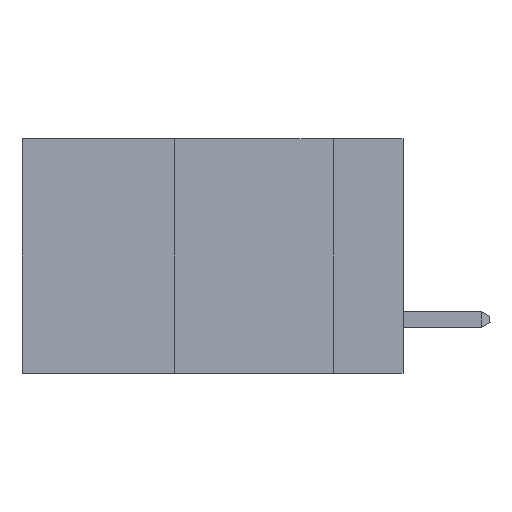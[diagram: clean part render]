
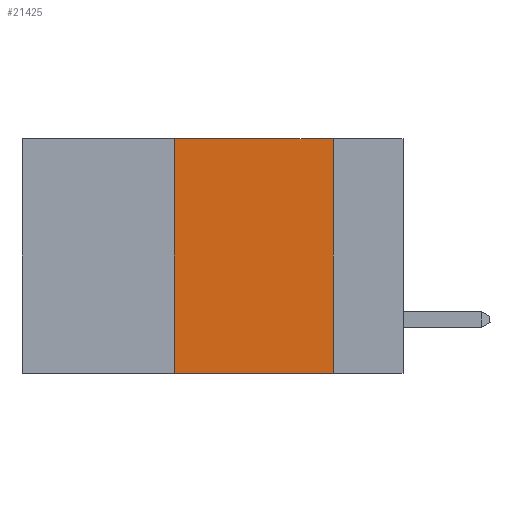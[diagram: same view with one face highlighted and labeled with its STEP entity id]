
A CAD part, left-side view. The second image highlights one B-rep face of the part: STEP entity #21425.
In plain terms, the highlighted planar face has unit normal (-1, 0, 0).
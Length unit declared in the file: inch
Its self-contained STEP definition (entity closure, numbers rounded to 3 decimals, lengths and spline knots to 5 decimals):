
#804 = LINE ( 'NONE', #48324, #30800 ) ;
#2694 = DIRECTION ( 'NONE',  ( 0., 0., -1. ) ) ;
#4091 = LINE ( 'NONE', #30993, #13079 ) ;
#6297 = CARTESIAN_POINT ( 'NONE',  ( 0., 0.36, -0.37 ) ) ;
#6637 = VERTEX_POINT ( 'NONE', #6297 ) ;
#9237 = VERTEX_POINT ( 'NONE', #23017 ) ;
#9293 = LINE ( 'NONE', #42395, #11704 ) ;
#9972 = EDGE_CURVE ( 'NONE', #19945, #35647, #4091, .T. ) ;
#10229 = CARTESIAN_POINT ( 'NONE',  ( 0., 0.11, 0. ) ) ;
#11704 = VECTOR ( 'NONE', #15233, 39.37008 ) ;
#13079 = VECTOR ( 'NONE', #39046, 39.37008 ) ;
#13133 = EDGE_CURVE ( 'NONE', #6637, #19945, #804, .T. ) ;
#14404 = EDGE_CURVE ( 'NONE', #35647, #9237, #40862, .T. ) ;
#14637 = EDGE_LOOP ( 'NONE', ( #26717, #46344, #33234, #18189 ) ) ;
#15233 = DIRECTION ( 'NONE',  ( 0., -1., 0. ) ) ;
#18189 = ORIENTED_EDGE ( 'NONE', *, *, #30617, .T. ) ;
#18473 = PLANE ( 'NONE',  #37638 ) ;
#19945 = VERTEX_POINT ( 'NONE', #43321 ) ;
#21425 = ADVANCED_FACE ( 'NONE', ( #24506 ), #18473, .F. ) ;
#22323 = DIRECTION ( 'NONE',  ( 0., 0., -1. ) ) ;
#23017 = CARTESIAN_POINT ( 'NONE',  ( 0., 0.11, -0.37 ) ) ;
#24506 = FACE_OUTER_BOUND ( 'NONE', #14637, .T. ) ;
#26717 = ORIENTED_EDGE ( 'NONE', *, *, #14404, .F. ) ;
#27049 = VECTOR ( 'NONE', #2694, 39.37008 ) ;
#30617 = EDGE_CURVE ( 'NONE', #6637, #9237, #9293, .T. ) ;
#30800 = VECTOR ( 'NONE', #44292, 39.37008 ) ;
#30993 = CARTESIAN_POINT ( 'NONE',  ( 0., 0.6, 0. ) ) ;
#33234 = ORIENTED_EDGE ( 'NONE', *, *, #13133, .F. ) ;
#33893 = DIRECTION ( 'NONE',  ( 1., 0., 0. ) ) ;
#35647 = VERTEX_POINT ( 'NONE', #48845 ) ;
#37638 = AXIS2_PLACEMENT_3D ( 'NONE', #45314, #33893, #22323 ) ;
#39046 = DIRECTION ( 'NONE',  ( 0., -1., 0. ) ) ;
#40862 = LINE ( 'NONE', #10229, #27049 ) ;
#42395 = CARTESIAN_POINT ( 'NONE',  ( 0., 0.6, -0.37 ) ) ;
#43321 = CARTESIAN_POINT ( 'NONE',  ( 0., 0.36, 0. ) ) ;
#44292 = DIRECTION ( 'NONE',  ( 0., 0., 1. ) ) ;
#45314 = CARTESIAN_POINT ( 'NONE',  ( 0., 0.6, 0. ) ) ;
#46344 = ORIENTED_EDGE ( 'NONE', *, *, #9972, .F. ) ;
#48324 = CARTESIAN_POINT ( 'NONE',  ( 0., 0.36, 0. ) ) ;
#48845 = CARTESIAN_POINT ( 'NONE',  ( 0., 0.11, 0. ) ) ;
